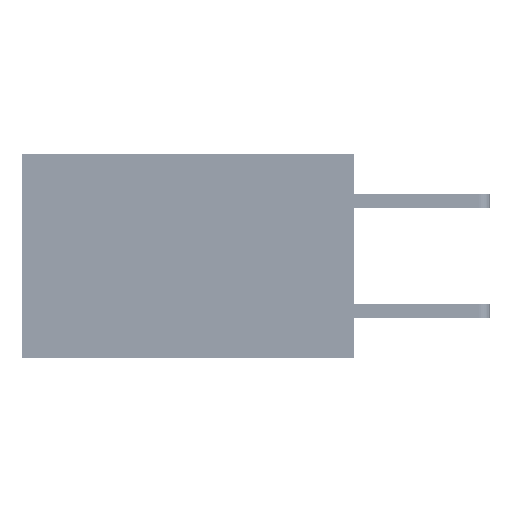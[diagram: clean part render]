
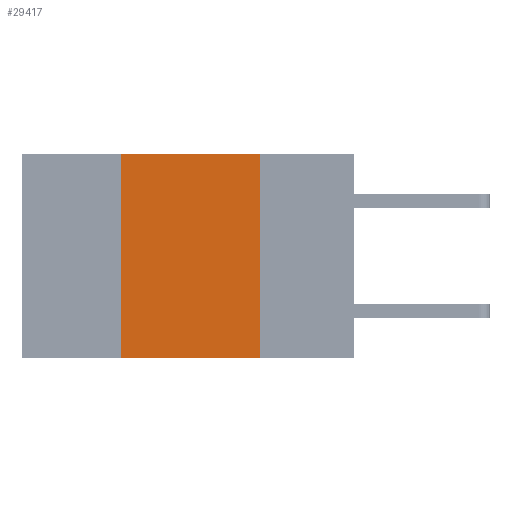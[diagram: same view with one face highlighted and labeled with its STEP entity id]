
A CAD part, left-side view. The second image highlights one B-rep face of the part: STEP entity #29417.
In plain terms, the highlighted planar face has unit normal (-1, 0, 0).
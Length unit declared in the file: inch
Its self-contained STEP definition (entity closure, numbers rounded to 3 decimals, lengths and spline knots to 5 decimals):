
#107 = PLANE ( 'NONE',  #34619 ) ;
#839 = CARTESIAN_POINT ( 'NONE',  ( 0., 0.17, 0. ) ) ;
#961 = EDGE_CURVE ( 'NONE', #31783, #13233, #23991, .T. ) ;
#2767 = DIRECTION ( 'NONE',  ( 0., -1., 0. ) ) ;
#3364 = LINE ( 'NONE', #3648, #7397 ) ;
#3482 = DIRECTION ( 'NONE',  ( 1., 0., 0. ) ) ;
#3648 = CARTESIAN_POINT ( 'NONE',  ( 0., 0.17, 0. ) ) ;
#3891 = LINE ( 'NONE', #23826, #36953 ) ;
#4027 = EDGE_LOOP ( 'NONE', ( #28164, #19481, #40436, #19851 ) ) ;
#7397 = VECTOR ( 'NONE', #10116, 39.37008 ) ;
#8157 = DIRECTION ( 'NONE',  ( 0., -1., 0. ) ) ;
#10116 = DIRECTION ( 'NONE',  ( 0., 0., -1. ) ) ;
#13233 = VERTEX_POINT ( 'NONE', #839 ) ;
#13534 = VERTEX_POINT ( 'NONE', #36933 ) ;
#19154 = CARTESIAN_POINT ( 'NONE',  ( 0., 0.6, 0. ) ) ;
#19481 = ORIENTED_EDGE ( 'NONE', *, *, #961, .F. ) ;
#19776 = CARTESIAN_POINT ( 'NONE',  ( 0., 0.42, 0. ) ) ;
#19851 = ORIENTED_EDGE ( 'NONE', *, *, #21895, .T. ) ;
#20453 = VECTOR ( 'NONE', #2767, 39.37008 ) ;
#21677 = EDGE_CURVE ( 'NONE', #32942, #31783, #40954, .T. ) ;
#21895 = EDGE_CURVE ( 'NONE', #32942, #13534, #3891, .T. ) ;
#22101 = EDGE_CURVE ( 'NONE', #13233, #13534, #3364, .T. ) ;
#22664 = CARTESIAN_POINT ( 'NONE',  ( 0., 0.6, 0. ) ) ;
#23826 = CARTESIAN_POINT ( 'NONE',  ( 0., 0.6, -0.37 ) ) ;
#23991 = LINE ( 'NONE', #19154, #20453 ) ;
#25887 = DIRECTION ( 'NONE',  ( 0., 0., -1. ) ) ;
#27077 = FACE_OUTER_BOUND ( 'NONE', #4027, .T. ) ;
#28164 = ORIENTED_EDGE ( 'NONE', *, *, #22101, .F. ) ;
#29417 = ADVANCED_FACE ( 'NONE', ( #27077 ), #107, .F. ) ;
#31783 = VERTEX_POINT ( 'NONE', #32569 ) ;
#32569 = CARTESIAN_POINT ( 'NONE',  ( 0., 0.42, 0. ) ) ;
#32858 = CARTESIAN_POINT ( 'NONE',  ( 0., 0.42, -0.37 ) ) ;
#32942 = VERTEX_POINT ( 'NONE', #32858 ) ;
#34619 = AXIS2_PLACEMENT_3D ( 'NONE', #22664, #3482, #25887 ) ;
#36311 = DIRECTION ( 'NONE',  ( 0., 0., 1. ) ) ;
#36933 = CARTESIAN_POINT ( 'NONE',  ( 0., 0.17, -0.37 ) ) ;
#36953 = VECTOR ( 'NONE', #8157, 39.37008 ) ;
#39965 = VECTOR ( 'NONE', #36311, 39.37008 ) ;
#40436 = ORIENTED_EDGE ( 'NONE', *, *, #21677, .F. ) ;
#40954 = LINE ( 'NONE', #19776, #39965 ) ;
